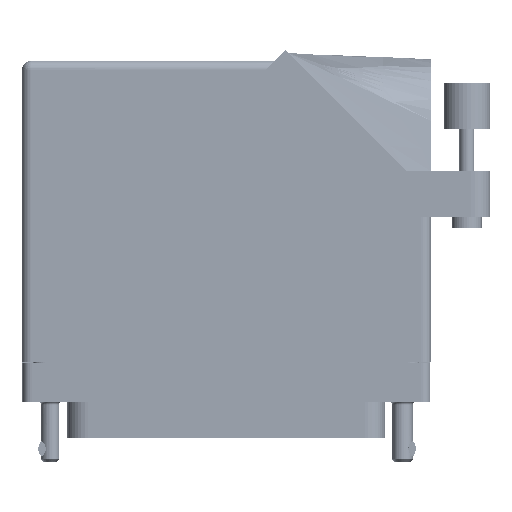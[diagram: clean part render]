
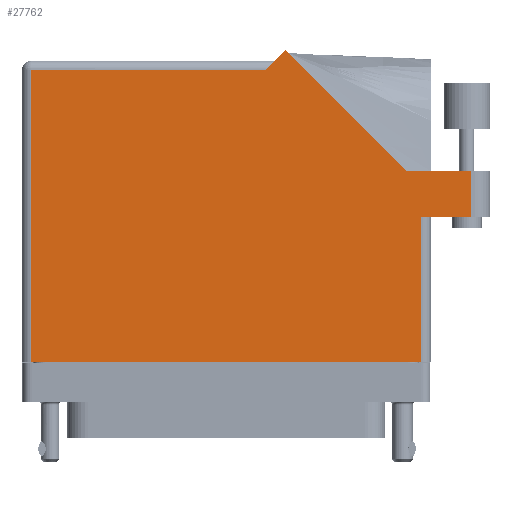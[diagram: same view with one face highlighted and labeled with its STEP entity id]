
A CAD part, front view. The second image highlights one B-rep face of the part: STEP entity #27762.
In plain terms, the highlighted face is planar.
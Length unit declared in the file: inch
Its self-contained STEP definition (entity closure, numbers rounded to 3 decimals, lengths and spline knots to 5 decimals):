
#2795 = CARTESIAN_POINT ( 'NONE',  ( -1.3775, 1.93, 0.765 ) ) ;
#3660 = VECTOR ( 'NONE', #8920, 39.37008 ) ;
#4237 = VECTOR ( 'NONE', #75349, 39.37008 ) ;
#5929 = ORIENTED_EDGE ( 'NONE', *, *, #89792, .T. ) ;
#6766 = EDGE_CURVE ( 'NONE', #29773, #77781, #92326, .T. ) ;
#8279 = VECTOR ( 'NONE', #20978, 39.37008 ) ;
#8920 = DIRECTION ( 'NONE',  ( -1., 0., 0. ) ) ;
#12925 = EDGE_CURVE ( 'NONE', #64860, #41702, #96225, .T. ) ;
#13595 = VERTEX_POINT ( 'NONE', #57924 ) ;
#14556 = LINE ( 'NONE', #52643, #8279 ) ;
#17012 = VERTEX_POINT ( 'NONE', #83219 ) ;
#19686 = VECTOR ( 'NONE', #52220, 39.37008 ) ;
#19778 = CARTESIAN_POINT ( 'NONE',  ( 1.21192, 1.187, 0.765 ) ) ;
#20046 = VECTOR ( 'NONE', #102068, 39.37008 ) ;
#20818 = CARTESIAN_POINT ( 'NONE',  ( 1.6525, 1.187, 0.765 ) ) ;
#20978 = DIRECTION ( 'NONE',  ( 1., 0., 0. ) ) ;
#23890 = LINE ( 'NONE', #95636, #52415 ) ;
#24590 = CARTESIAN_POINT ( 'NONE',  ( 1.6525, 0.88, 0.765 ) ) ;
#24923 = CARTESIAN_POINT ( 'NONE',  ( 1.7775, 1.187, 0.765 ) ) ;
#27762 = ADVANCED_FACE ( 'NONE', ( #88686 ), #88929, .F. ) ;
#29119 = CARTESIAN_POINT ( 'NONE',  ( 0.39821, 2.00071, 0.765 ) ) ;
#29773 = VERTEX_POINT ( 'NONE', #24590 ) ;
#30568 = LINE ( 'NONE', #50184, #47997 ) ;
#34771 = LINE ( 'NONE', #24923, #3660 ) ;
#34856 = CARTESIAN_POINT ( 'NONE',  ( -1.3155, -0.1, 0.765 ) ) ;
#36888 = ORIENTED_EDGE ( 'NONE', *, *, #82004, .T. ) ;
#37600 = CARTESIAN_POINT ( 'NONE',  ( 1.3155, 0.88, 0.765 ) ) ;
#38231 = EDGE_LOOP ( 'NONE', ( #36888, #70072, #90758, #78872, #98138, #5929, #74602, #40473, #50759 ) ) ;
#38655 = CARTESIAN_POINT ( 'NONE',  ( 1.6525, 1.187, 0.765 ) ) ;
#40080 = VERTEX_POINT ( 'NONE', #37600 ) ;
#40473 = ORIENTED_EDGE ( 'NONE', *, *, #59257, .T. ) ;
#40797 = LINE ( 'NONE', #34856, #19686 ) ;
#41178 = LINE ( 'NONE', #71496, #20046 ) ;
#41702 = VERTEX_POINT ( 'NONE', #29119 ) ;
#46707 = EDGE_CURVE ( 'NONE', #77781, #64860, #34771, .T. ) ;
#47997 = VECTOR ( 'NONE', #89419, 39.37008 ) ;
#48058 = DIRECTION ( 'NONE',  ( -0.707, -0.707, 0. ) ) ;
#49350 = VERTEX_POINT ( 'NONE', #88062 ) ;
#50123 = VERTEX_POINT ( 'NONE', #81658 ) ;
#50184 = CARTESIAN_POINT ( 'NONE',  ( 1.3155, 0.88, 0.765 ) ) ;
#50377 = DIRECTION ( 'NONE',  ( 0., 0., -1. ) ) ;
#50759 = ORIENTED_EDGE ( 'NONE', *, *, #83483, .T. ) ;
#51201 = CARTESIAN_POINT ( 'NONE',  ( 1.21192, 1.187, 0.765 ) ) ;
#52220 = DIRECTION ( 'NONE',  ( 0., -1., 0. ) ) ;
#52415 = VECTOR ( 'NONE', #48058, 39.37008 ) ;
#52643 = CARTESIAN_POINT ( 'NONE',  ( 1.3775, 0.88, 0.765 ) ) ;
#55770 = DIRECTION ( 'NONE',  ( 1., 0., 0. ) ) ;
#57924 = CARTESIAN_POINT ( 'NONE',  ( 1.3155, -0.1, 0.765 ) ) ;
#59257 = EDGE_CURVE ( 'NONE', #17012, #13595, #101708, .T. ) ;
#59494 = VECTOR ( 'NONE', #55770, 39.37008 ) ;
#59521 = EDGE_CURVE ( 'NONE', #50123, #17012, #40797, .T. ) ;
#64860 = VERTEX_POINT ( 'NONE', #51201 ) ;
#70072 = ORIENTED_EDGE ( 'NONE', *, *, #6766, .T. ) ;
#71196 = VECTOR ( 'NONE', #77236, 39.37008 ) ;
#71496 = CARTESIAN_POINT ( 'NONE',  ( -1.3775, 1.868, 0.765 ) ) ;
#74602 = ORIENTED_EDGE ( 'NONE', *, *, #59521, .T. ) ;
#75349 = DIRECTION ( 'NONE',  ( -0.707, 0.707, 0. ) ) ;
#77236 = DIRECTION ( 'NONE',  ( 0., 1., 0. ) ) ;
#77781 = VERTEX_POINT ( 'NONE', #20818 ) ;
#78872 = ORIENTED_EDGE ( 'NONE', *, *, #12925, .T. ) ;
#79676 = CARTESIAN_POINT ( 'NONE',  ( -1.3775, -0.1, 0.765 ) ) ;
#81658 = CARTESIAN_POINT ( 'NONE',  ( -1.3155, 1.868, 0.765 ) ) ;
#82004 = EDGE_CURVE ( 'NONE', #40080, #29773, #14556, .T. ) ;
#83219 = CARTESIAN_POINT ( 'NONE',  ( -1.3155, -0.1, 0.765 ) ) ;
#83483 = EDGE_CURVE ( 'NONE', #13595, #40080, #30568, .T. ) ;
#85985 = AXIS2_PLACEMENT_3D ( 'NONE', #2795, #50377, #89946 ) ;
#88062 = CARTESIAN_POINT ( 'NONE',  ( 0.2655, 1.868, 0.765 ) ) ;
#88686 = FACE_OUTER_BOUND ( 'NONE', #38231, .T. ) ;
#88929 = PLANE ( 'NONE',  #85985 ) ;
#89419 = DIRECTION ( 'NONE',  ( 0., 1., 0. ) ) ;
#89792 = EDGE_CURVE ( 'NONE', #49350, #50123, #41178, .T. ) ;
#89946 = DIRECTION ( 'NONE',  ( -1., 0., 0. ) ) ;
#90758 = ORIENTED_EDGE ( 'NONE', *, *, #46707, .T. ) ;
#92326 = LINE ( 'NONE', #38655, #71196 ) ;
#95636 = CARTESIAN_POINT ( 'NONE',  ( 0.3275, 1.93, 0.765 ) ) ;
#96225 = LINE ( 'NONE', #19778, #4237 ) ;
#98138 = ORIENTED_EDGE ( 'NONE', *, *, #99041, .T. ) ;
#99041 = EDGE_CURVE ( 'NONE', #41702, #49350, #23890, .T. ) ;
#101708 = LINE ( 'NONE', #79676, #59494 ) ;
#102068 = DIRECTION ( 'NONE',  ( -1., 0., 0. ) ) ;
